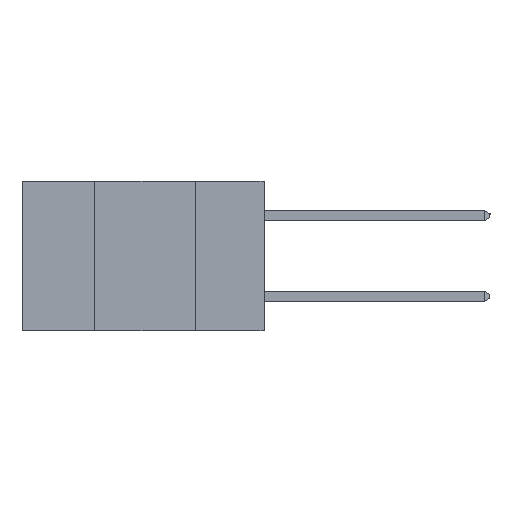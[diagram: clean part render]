
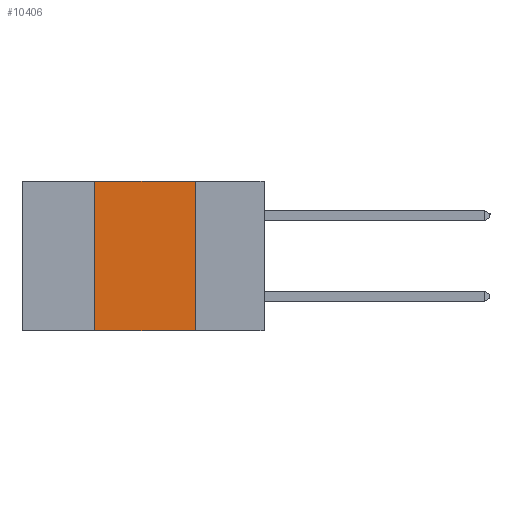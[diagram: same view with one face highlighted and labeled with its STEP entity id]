
A CAD part, left-side view. The second image highlights one B-rep face of the part: STEP entity #10406.
In plain terms, the highlighted planar face has unit normal (-1, 0, 0).
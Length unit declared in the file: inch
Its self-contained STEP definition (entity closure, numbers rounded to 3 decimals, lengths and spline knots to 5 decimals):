
#366 = CARTESIAN_POINT ( 'NONE',  ( 0., 0.17, -0.37 ) ) ;
#418 = AXIS2_PLACEMENT_3D ( 'NONE', #5518, #6859, #7804 ) ;
#520 = DIRECTION ( 'NONE',  ( 0., 0., -1. ) ) ;
#563 = VERTEX_POINT ( 'NONE', #6887 ) ;
#682 = VECTOR ( 'NONE', #12154, 39.37008 ) ;
#790 = CARTESIAN_POINT ( 'NONE',  ( 0., 0.17, -0.37 ) ) ;
#1755 = DIRECTION ( 'NONE',  ( 0., -1., 0. ) ) ;
#2390 = VECTOR ( 'NONE', #1755, 39.37008 ) ;
#3001 = PLANE ( 'NONE',  #418 ) ;
#3078 = FACE_OUTER_BOUND ( 'NONE', #9511, .T. ) ;
#4195 = CARTESIAN_POINT ( 'NONE',  ( 0., 0.42, -0.37 ) ) ;
#4354 = LINE ( 'NONE', #8993, #2390 ) ;
#4675 = ORIENTED_EDGE ( 'NONE', *, *, #5780, .F. ) ;
#4708 = VERTEX_POINT ( 'NONE', #13370 ) ;
#5518 = CARTESIAN_POINT ( 'NONE',  ( 0., 0.6, 0. ) ) ;
#5780 = EDGE_CURVE ( 'NONE', #9289, #4708, #14951, .T. ) ;
#6436 = CARTESIAN_POINT ( 'NONE',  ( 0., 0.42, -0.37 ) ) ;
#6859 = DIRECTION ( 'NONE',  ( 1., 0., 0. ) ) ;
#6887 = CARTESIAN_POINT ( 'NONE',  ( 0., 0.17, 0. ) ) ;
#7161 = VECTOR ( 'NONE', #520, 39.37008 ) ;
#7527 = LINE ( 'NONE', #8476, #682 ) ;
#7804 = DIRECTION ( 'NONE',  ( 0., 0., -1. ) ) ;
#8476 = CARTESIAN_POINT ( 'NONE',  ( 0., 0.6, 0. ) ) ;
#8985 = DIRECTION ( 'NONE',  ( 0., 0., 1. ) ) ;
#8993 = CARTESIAN_POINT ( 'NONE',  ( 0., 0.6, -0.37 ) ) ;
#9289 = VERTEX_POINT ( 'NONE', #6436 ) ;
#9511 = EDGE_LOOP ( 'NONE', ( #14849, #9673, #4675, #11348 ) ) ;
#9673 = ORIENTED_EDGE ( 'NONE', *, *, #12915, .F. ) ;
#10406 = ADVANCED_FACE ( 'NONE', ( #3078 ), #3001, .F. ) ;
#11348 = ORIENTED_EDGE ( 'NONE', *, *, #15432, .T. ) ;
#12154 = DIRECTION ( 'NONE',  ( 0., -1., 0. ) ) ;
#12343 = VERTEX_POINT ( 'NONE', #790 ) ;
#12915 = EDGE_CURVE ( 'NONE', #4708, #563, #7527, .T. ) ;
#13360 = VECTOR ( 'NONE', #8985, 39.37008 ) ;
#13370 = CARTESIAN_POINT ( 'NONE',  ( 0., 0.42, 0. ) ) ;
#14669 = LINE ( 'NONE', #366, #7161 ) ;
#14784 = EDGE_CURVE ( 'NONE', #563, #12343, #14669, .T. ) ;
#14849 = ORIENTED_EDGE ( 'NONE', *, *, #14784, .F. ) ;
#14951 = LINE ( 'NONE', #4195, #13360 ) ;
#15432 = EDGE_CURVE ( 'NONE', #9289, #12343, #4354, .T. ) ;
